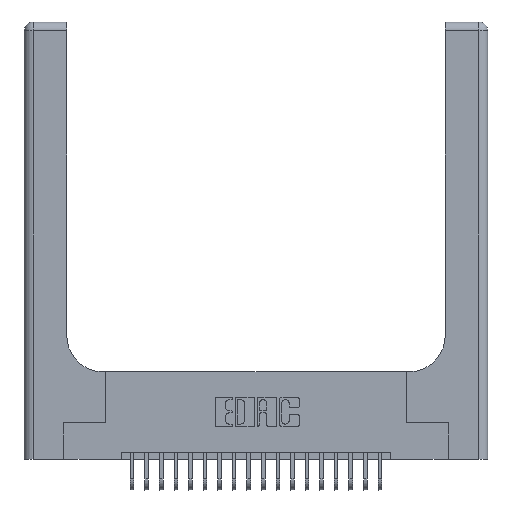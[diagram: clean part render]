
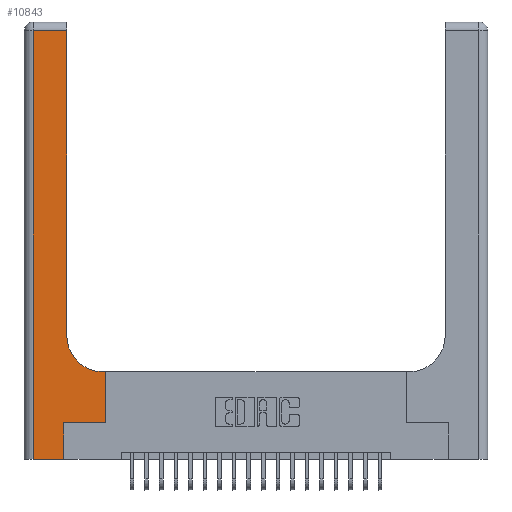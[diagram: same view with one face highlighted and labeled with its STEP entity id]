
A CAD part, top view. The second image highlights one B-rep face of the part: STEP entity #10843.
In plain terms, the highlighted planar face has unit normal (0, 0, 1).
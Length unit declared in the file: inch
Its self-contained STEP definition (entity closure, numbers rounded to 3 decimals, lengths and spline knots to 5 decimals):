
#471 = EDGE_CURVE ( 'NONE', #2064, #21728, #22142, .T. ) ;
#508 = ORIENTED_EDGE ( 'NONE', *, *, #1574, .T. ) ;
#754 = DIRECTION ( 'NONE',  ( 0., -1., 0. ) ) ;
#787 = CARTESIAN_POINT ( 'NONE',  ( 0.06, 3., 0.37 ) ) ;
#1574 = EDGE_CURVE ( 'NONE', #20272, #8111, #19830, .T. ) ;
#1711 = CARTESIAN_POINT ( 'NONE',  ( 0.5585, 0.25, 0.37 ) ) ;
#1747 = DIRECTION ( 'NONE',  ( 0., 0., -1. ) ) ;
#2064 = VERTEX_POINT ( 'NONE', #14546 ) ;
#2373 = EDGE_CURVE ( 'NONE', #15560, #7315, #24013, .T. ) ;
#2593 = ORIENTED_EDGE ( 'NONE', *, *, #4800, .T. ) ;
#3252 = CARTESIAN_POINT ( 'NONE',  ( 0.2915, 0.85, 0.37 ) ) ;
#3700 = CARTESIAN_POINT ( 'NONE',  ( 0.5585, 0.25, 0.37 ) ) ;
#4364 = EDGE_CURVE ( 'NONE', #9570, #8898, #5485, .T. ) ;
#4649 = CARTESIAN_POINT ( 'NONE',  ( 0.269, 0.25, 0.37 ) ) ;
#4800 = EDGE_CURVE ( 'NONE', #8898, #19381, #16066, .T. ) ;
#4936 = VECTOR ( 'NONE', #11818, 39.37008 ) ;
#5216 = LINE ( 'NONE', #23158, #10171 ) ;
#5485 = LINE ( 'NONE', #1711, #19741 ) ;
#5705 = DIRECTION ( 'NONE',  ( 0., 1., 0. ) ) ;
#5906 = CARTESIAN_POINT ( 'NONE',  ( 0.5415, 0.85, 0.37 ) ) ;
#6547 = EDGE_CURVE ( 'NONE', #21728, #9570, #16036, .T. ) ;
#6764 = CARTESIAN_POINT ( 'NONE',  ( 0.2915, 0.6, 0.37 ) ) ;
#7179 = CARTESIAN_POINT ( 'NONE',  ( 0., 0., 0.37 ) ) ;
#7296 = ORIENTED_EDGE ( 'NONE', *, *, #22334, .T. ) ;
#7315 = VERTEX_POINT ( 'NONE', #10673 ) ;
#7729 = CARTESIAN_POINT ( 'NONE',  ( 0.5415, 0.6, 0.37 ) ) ;
#7827 = DIRECTION ( 'NONE',  ( 1., 0., 0. ) ) ;
#7880 = AXIS2_PLACEMENT_3D ( 'NONE', #5906, #18945, #7827 ) ;
#8030 = VECTOR ( 'NONE', #14885, 39.37008 ) ;
#8111 = VERTEX_POINT ( 'NONE', #23841 ) ;
#8169 = LINE ( 'NONE', #7179, #12594 ) ;
#8226 = FACE_OUTER_BOUND ( 'NONE', #14468, .T. ) ;
#8898 = VERTEX_POINT ( 'NONE', #14884 ) ;
#9098 = DIRECTION ( 'NONE',  ( 1., 0., 0. ) ) ;
#9231 = CARTESIAN_POINT ( 'NONE',  ( 0.06, 2.94, 0.37 ) ) ;
#9315 = CARTESIAN_POINT ( 'NONE',  ( 0.2915, 3., 0.37 ) ) ;
#9570 = VERTEX_POINT ( 'NONE', #3700 ) ;
#10171 = VECTOR ( 'NONE', #12305, 39.37008 ) ;
#10499 = EDGE_CURVE ( 'NONE', #7315, #20272, #5216, .T. ) ;
#10673 = CARTESIAN_POINT ( 'NONE',  ( 0.2915, 2.94, 0.37 ) ) ;
#10843 = ADVANCED_FACE ( 'NONE', ( #8226 ), #24078, .F. ) ;
#11266 = ORIENTED_EDGE ( 'NONE', *, *, #471, .T. ) ;
#11368 = CARTESIAN_POINT ( 'NONE',  ( 0., 3., 0.37 ) ) ;
#11581 = ORIENTED_EDGE ( 'NONE', *, *, #6547, .T. ) ;
#11818 = DIRECTION ( 'NONE',  ( 0., 1., 0. ) ) ;
#12305 = DIRECTION ( 'NONE',  ( -1., 0., 0. ) ) ;
#12594 = VECTOR ( 'NONE', #9098, 39.37008 ) ;
#12854 = AXIS2_PLACEMENT_3D ( 'NONE', #11368, #1747, #15127 ) ;
#13723 = ORIENTED_EDGE ( 'NONE', *, *, #23863, .T. ) ;
#13810 = CARTESIAN_POINT ( 'NONE',  ( 0.269, 0.25, 0.37 ) ) ;
#14468 = EDGE_LOOP ( 'NONE', ( #22947, #15733, #508, #13723, #11266, #11581, #18113, #2593, #7296 ) ) ;
#14546 = CARTESIAN_POINT ( 'NONE',  ( 0.269, 0., 0.37 ) ) ;
#14677 = CARTESIAN_POINT ( 'NONE',  ( 0.269, 0., 0.37 ) ) ;
#14884 = CARTESIAN_POINT ( 'NONE',  ( 0.5585, 0.6, 0.37 ) ) ;
#14885 = DIRECTION ( 'NONE',  ( 0., 1., 0. ) ) ;
#15127 = DIRECTION ( 'NONE',  ( -1., 0., 0. ) ) ;
#15560 = VERTEX_POINT ( 'NONE', #3252 ) ;
#15674 = DIRECTION ( 'NONE',  ( 1., 0., 0. ) ) ;
#15733 = ORIENTED_EDGE ( 'NONE', *, *, #10499, .T. ) ;
#16036 = LINE ( 'NONE', #13810, #20271 ) ;
#16066 = LINE ( 'NONE', #6764, #21422 ) ;
#16120 = DIRECTION ( 'NONE',  ( -1., 0., 0. ) ) ;
#18113 = ORIENTED_EDGE ( 'NONE', *, *, #4364, .T. ) ;
#18945 = DIRECTION ( 'NONE',  ( 0., 0., -1. ) ) ;
#19381 = VERTEX_POINT ( 'NONE', #7729 ) ;
#19741 = VECTOR ( 'NONE', #5705, 39.37008 ) ;
#19830 = LINE ( 'NONE', #787, #20420 ) ;
#20271 = VECTOR ( 'NONE', #15674, 39.37008 ) ;
#20272 = VERTEX_POINT ( 'NONE', #9231 ) ;
#20420 = VECTOR ( 'NONE', #754, 39.37008 ) ;
#21422 = VECTOR ( 'NONE', #16120, 39.37008 ) ;
#21728 = VERTEX_POINT ( 'NONE', #4649 ) ;
#22142 = LINE ( 'NONE', #14677, #8030 ) ;
#22334 = EDGE_CURVE ( 'NONE', #19381, #15560, #22616, .T. ) ;
#22616 = CIRCLE ( 'NONE', #7880, 0.25 ) ;
#22947 = ORIENTED_EDGE ( 'NONE', *, *, #2373, .T. ) ;
#23158 = CARTESIAN_POINT ( 'NONE',  ( 0., 2.94, 0.37 ) ) ;
#23841 = CARTESIAN_POINT ( 'NONE',  ( 0.06, 0., 0.37 ) ) ;
#23863 = EDGE_CURVE ( 'NONE', #8111, #2064, #8169, .T. ) ;
#24013 = LINE ( 'NONE', #9315, #4936 ) ;
#24078 = PLANE ( 'NONE',  #12854 ) ;
